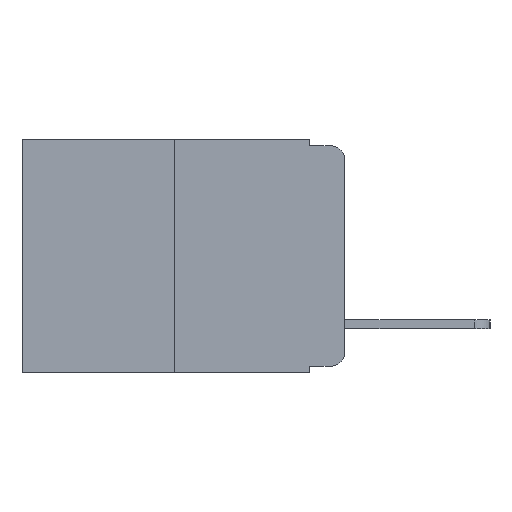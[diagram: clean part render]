
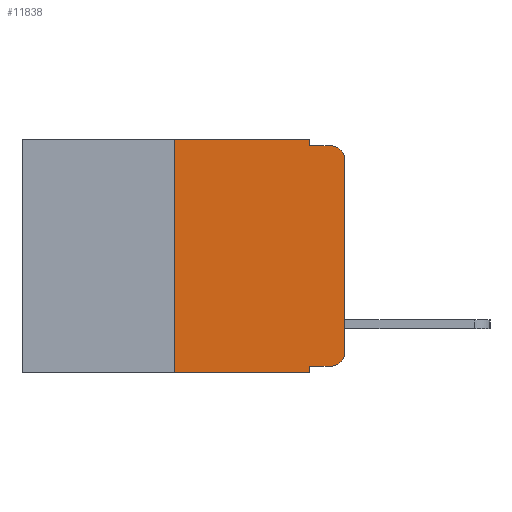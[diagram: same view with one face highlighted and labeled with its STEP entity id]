
A CAD part, left-side view. The second image highlights one B-rep face of the part: STEP entity #11838.
In plain terms, the highlighted planar face has unit normal (-1, 0, 0).
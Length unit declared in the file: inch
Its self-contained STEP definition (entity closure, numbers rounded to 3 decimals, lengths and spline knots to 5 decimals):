
#83 = EDGE_CURVE ( 'NONE', #6243, #13971, #13480, .T. ) ;
#284 = CARTESIAN_POINT ( 'NONE',  ( 0., 0.02, -0.03 ) ) ;
#963 = EDGE_CURVE ( 'NONE', #1061, #6243, #18363, .T. ) ;
#1019 = ORIENTED_EDGE ( 'NONE', *, *, #8761, .T. ) ;
#1051 = DIRECTION ( 'NONE',  ( 0., -1., 0. ) ) ;
#1061 = VERTEX_POINT ( 'NONE', #12979 ) ;
#1297 = EDGE_CURVE ( 'NONE', #9826, #7199, #16722, .T. ) ;
#1404 = CARTESIAN_POINT ( 'NONE',  ( 0., 0.051, 0. ) ) ;
#1991 = DIRECTION ( 'NONE',  ( 0., 0., -1. ) ) ;
#2097 = VERTEX_POINT ( 'NONE', #4671 ) ;
#2826 = CIRCLE ( 'NONE', #19057, 0.02 ) ;
#3145 = CARTESIAN_POINT ( 'NONE',  ( 0., 0.051, -0.01 ) ) ;
#3377 = DIRECTION ( 'NONE',  ( 0., 0., -1. ) ) ;
#3479 = DIRECTION ( 'NONE',  ( 0., -1., 0. ) ) ;
#3735 = DIRECTION ( 'NONE',  ( 0., 0., -1. ) ) ;
#3895 = CARTESIAN_POINT ( 'NONE',  ( 0., 0.051, -0.333 ) ) ;
#3903 = CARTESIAN_POINT ( 'NONE',  ( 0., 0.051, -0.01 ) ) ;
#4182 = DIRECTION ( 'NONE',  ( 1., 0., 0. ) ) ;
#4270 = EDGE_LOOP ( 'NONE', ( #17086, #1019, #14050, #14507, #6864, #18948, #11895, #15920, #12388, #12860 ) ) ;
#4292 = LINE ( 'NONE', #17132, #20091 ) ;
#4307 = PLANE ( 'NONE',  #5293 ) ;
#4671 = CARTESIAN_POINT ( 'NONE',  ( 0., 0., -0.03 ) ) ;
#5238 = VECTOR ( 'NONE', #3377, 39.37008 ) ;
#5293 = AXIS2_PLACEMENT_3D ( 'NONE', #19440, #4182, #15000 ) ;
#5487 = LINE ( 'NONE', #17932, #6005 ) ;
#5556 = EDGE_CURVE ( 'NONE', #13971, #13801, #13434, .T. ) ;
#5927 = CARTESIAN_POINT ( 'NONE',  ( 0., 0.051, -0.333 ) ) ;
#5976 = CARTESIAN_POINT ( 'NONE',  ( 0., 0.051, 0. ) ) ;
#6005 = VECTOR ( 'NONE', #19442, 39.37008 ) ;
#6110 = CARTESIAN_POINT ( 'NONE',  ( 0., 0.02, -0.313 ) ) ;
#6231 = VECTOR ( 'NONE', #3479, 39.37008 ) ;
#6243 = VERTEX_POINT ( 'NONE', #5976 ) ;
#6864 = ORIENTED_EDGE ( 'NONE', *, *, #963, .F. ) ;
#7082 = VECTOR ( 'NONE', #1051, 39.37008 ) ;
#7199 = VERTEX_POINT ( 'NONE', #11371 ) ;
#7344 = VERTEX_POINT ( 'NONE', #11632 ) ;
#7505 = DIRECTION ( 'NONE',  ( 0., -1., 0. ) ) ;
#7559 = FACE_OUTER_BOUND ( 'NONE', #4270, .T. ) ;
#7722 = DIRECTION ( 'NONE',  ( 0., 0., -1. ) ) ;
#8761 = EDGE_CURVE ( 'NONE', #2097, #13801, #2826, .T. ) ;
#8871 = VERTEX_POINT ( 'NONE', #3895 ) ;
#8932 = VECTOR ( 'NONE', #14019, 39.37008 ) ;
#9787 = EDGE_CURVE ( 'NONE', #12728, #2097, #4292, .T. ) ;
#9826 = VERTEX_POINT ( 'NONE', #14321 ) ;
#11261 = CARTESIAN_POINT ( 'NONE',  ( 0., 0.473, 0. ) ) ;
#11371 = CARTESIAN_POINT ( 'NONE',  ( 0., 0.051, -0.343 ) ) ;
#11416 = DIRECTION ( 'NONE',  ( -1., 0., 0. ) ) ;
#11632 = CARTESIAN_POINT ( 'NONE',  ( 0., 0.02, -0.333 ) ) ;
#11838 = ADVANCED_FACE ( 'NONE', ( #7559 ), #4307, .F. ) ;
#11895 = ORIENTED_EDGE ( 'NONE', *, *, #1297, .T. ) ;
#12388 = ORIENTED_EDGE ( 'NONE', *, *, #17227, .T. ) ;
#12727 = VECTOR ( 'NONE', #7505, 39.37008 ) ;
#12728 = VERTEX_POINT ( 'NONE', #18627 ) ;
#12860 = ORIENTED_EDGE ( 'NONE', *, *, #13191, .T. ) ;
#12979 = CARTESIAN_POINT ( 'NONE',  ( 0., 0.25, 0. ) ) ;
#13191 = EDGE_CURVE ( 'NONE', #7344, #12728, #13967, .T. ) ;
#13434 = LINE ( 'NONE', #3145, #8932 ) ;
#13480 = LINE ( 'NONE', #1404, #5238 ) ;
#13801 = VERTEX_POINT ( 'NONE', #17290 ) ;
#13967 = CIRCLE ( 'NONE', #15387, 0.02 ) ;
#13971 = VERTEX_POINT ( 'NONE', #3903 ) ;
#14019 = DIRECTION ( 'NONE',  ( 0., -1., 0. ) ) ;
#14050 = ORIENTED_EDGE ( 'NONE', *, *, #5556, .F. ) ;
#14189 = DIRECTION ( 'NONE',  ( 0., 0., 1. ) ) ;
#14321 = CARTESIAN_POINT ( 'NONE',  ( 0., 0.25, -0.343 ) ) ;
#14507 = ORIENTED_EDGE ( 'NONE', *, *, #83, .F. ) ;
#15000 = DIRECTION ( 'NONE',  ( 0., 0., -1. ) ) ;
#15079 = CARTESIAN_POINT ( 'NONE',  ( 0., 0.473, -0.343 ) ) ;
#15187 = LINE ( 'NONE', #5927, #7082 ) ;
#15387 = AXIS2_PLACEMENT_3D ( 'NONE', #6110, #16791, #7722 ) ;
#15920 = ORIENTED_EDGE ( 'NONE', *, *, #18227, .F. ) ;
#16306 = LINE ( 'NONE', #17514, #19817 ) ;
#16722 = LINE ( 'NONE', #15079, #12727 ) ;
#16791 = DIRECTION ( 'NONE',  ( -1., 0., 0. ) ) ;
#17086 = ORIENTED_EDGE ( 'NONE', *, *, #9787, .T. ) ;
#17132 = CARTESIAN_POINT ( 'NONE',  ( 0., 0., 0. ) ) ;
#17227 = EDGE_CURVE ( 'NONE', #8871, #7344, #15187, .T. ) ;
#17290 = CARTESIAN_POINT ( 'NONE',  ( 0., 0.02, -0.01 ) ) ;
#17514 = CARTESIAN_POINT ( 'NONE',  ( 0., 0.051, 0. ) ) ;
#17932 = CARTESIAN_POINT ( 'NONE',  ( 0., 0.25, 0. ) ) ;
#18227 = EDGE_CURVE ( 'NONE', #8871, #7199, #16306, .T. ) ;
#18363 = LINE ( 'NONE', #11261, #6231 ) ;
#18627 = CARTESIAN_POINT ( 'NONE',  ( 0., 0., -0.313 ) ) ;
#18948 = ORIENTED_EDGE ( 'NONE', *, *, #19222, .F. ) ;
#19057 = AXIS2_PLACEMENT_3D ( 'NONE', #284, #11416, #1991 ) ;
#19222 = EDGE_CURVE ( 'NONE', #9826, #1061, #5487, .T. ) ;
#19440 = CARTESIAN_POINT ( 'NONE',  ( 0., 0.473, 0. ) ) ;
#19442 = DIRECTION ( 'NONE',  ( 0., 0., 1. ) ) ;
#19817 = VECTOR ( 'NONE', #3735, 39.37008 ) ;
#20091 = VECTOR ( 'NONE', #14189, 39.37008 ) ;
